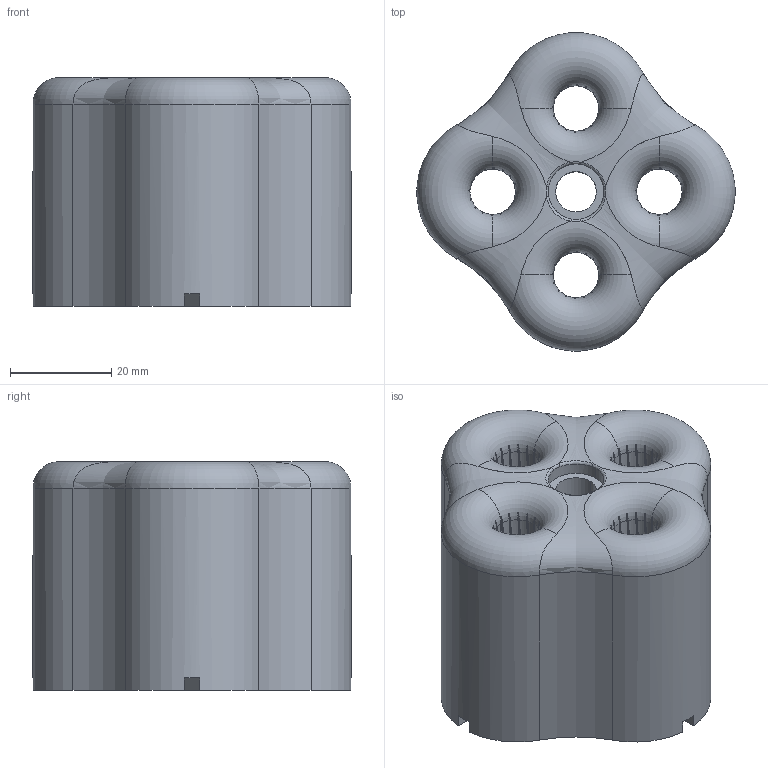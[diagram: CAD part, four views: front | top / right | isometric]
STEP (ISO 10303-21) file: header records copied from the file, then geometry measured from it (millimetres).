
FILE_DESCRIPTION (( 'STEP AP214' ), '1' );
FILE_NAME ('Barrel.STEP', '2013-11-21T02:34:40', ( '' ), ( '' ), 'SwSTEP 2.0', 'SolidWorks 2013', '' );
FILE_SCHEMA (( 'AUTOMOTIVE_DESIGN' ));
Length unit declared in the file: millimetre
Products named in the file (1): Barrel
Bounding box: 62.93 x 62.93 x 45.24 mm (x, y, z)
Volume: 98889.6 mm3; surface area: 19321.7 mm2
Topology: 1 solids, 1 shells, 1154 faces, 2800 edges, 1516 vertices
Faces by surface type: bspline 972, cylinder 88, torus 72, plane 14, cone 8
Entity records: 70470 total; most frequent: CARTESIAN_POINT 51213, ORIENTED_EDGE 5344, EDGE_CURVE 2672, DIRECTION 2222, B_SPLINE_CURVE_WITH_KNOTS 1710, VERTEX_POINT 1516, EDGE_LOOP 1160, FACE_OUTER_BOUND 1154
